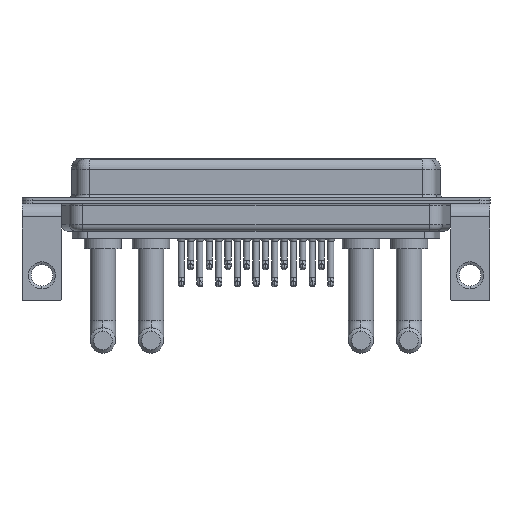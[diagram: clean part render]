
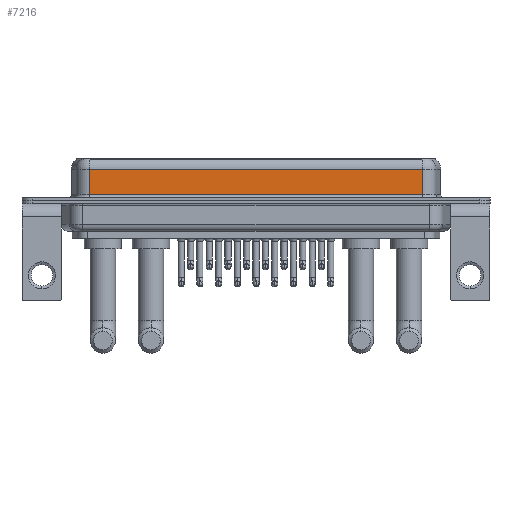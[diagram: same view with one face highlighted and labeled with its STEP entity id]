
A CAD part, front view. The second image highlights one B-rep face of the part: STEP entity #7216.
In plain terms, the highlighted planar face has unit normal (0, -1, 0).
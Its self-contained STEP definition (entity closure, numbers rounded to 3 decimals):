
#426 = EDGE_CURVE ( 'NONE', #21630, #22538, #20422, .T. ) ;
#877 = ORIENTED_EDGE ( 'NONE', *, *, #426, .T. ) ;
#1028 = VECTOR ( 'NONE', #13619, 1000. ) ;
#1091 = CARTESIAN_POINT ( 'NONE',  ( 56.462, -3.95, 6.4 ) ) ;
#1149 = LINE ( 'NONE', #15602, #1028 ) ;
#1449 = AXIS2_PLACEMENT_3D ( 'NONE', #1091, #13446, #4660 ) ;
#4433 = VECTOR ( 'NONE', #10505, 1000. ) ;
#4660 = DIRECTION ( 'NONE',  ( 0., 0., 1. ) ) ;
#4919 = EDGE_CURVE ( 'NONE', #10563, #21630, #1149, .T. ) ;
#4928 = ORIENTED_EDGE ( 'NONE', *, *, #17255, .F. ) ;
#5510 = ORIENTED_EDGE ( 'NONE', *, *, #4919, .T. ) ;
#6090 = ORIENTED_EDGE ( 'NONE', *, *, #15577, .T. ) ;
#6255 = VECTOR ( 'NONE', #6483, 1000. ) ;
#6483 = DIRECTION ( 'NONE',  ( 1., 0., 0. ) ) ;
#7216 = ADVANCED_FACE ( 'NONE', ( #20575 ), #11484, .F. ) ;
#8173 = DIRECTION ( 'NONE',  ( 0., 0., -1. ) ) ;
#8788 = VERTEX_POINT ( 'NONE', #19651 ) ;
#8938 = VECTOR ( 'NONE', #8173, 1000. ) ;
#9002 = CARTESIAN_POINT ( 'NONE',  ( 56.462, -3.95, 4.65 ) ) ;
#9912 = LINE ( 'NONE', #16959, #8938 ) ;
#10505 = DIRECTION ( 'NONE',  ( -1., 0., 0. ) ) ;
#10563 = VERTEX_POINT ( 'NONE', #21608 ) ;
#11484 = PLANE ( 'NONE',  #1449 ) ;
#13446 = DIRECTION ( 'NONE',  ( 0., 1., 0. ) ) ;
#13619 = DIRECTION ( 'NONE',  ( 0., 0., -1. ) ) ;
#14200 = LINE ( 'NONE', #9002, #4433 ) ;
#14253 = CARTESIAN_POINT ( 'NONE',  ( 56.462, -3.95, 0.9 ) ) ;
#15577 = EDGE_CURVE ( 'NONE', #8788, #10563, #14200, .T. ) ;
#15602 = CARTESIAN_POINT ( 'NONE',  ( 7.038, -3.95, 6.4 ) ) ;
#16959 = CARTESIAN_POINT ( 'NONE',  ( 56.462, -3.95, 6.4 ) ) ;
#17255 = EDGE_CURVE ( 'NONE', #8788, #22538, #9912, .T. ) ;
#18270 = EDGE_LOOP ( 'NONE', ( #4928, #6090, #5510, #877 ) ) ;
#19651 = CARTESIAN_POINT ( 'NONE',  ( 56.462, -3.95, 4.65 ) ) ;
#20422 = LINE ( 'NONE', #22267, #6255 ) ;
#20575 = FACE_OUTER_BOUND ( 'NONE', #18270, .T. ) ;
#21554 = CARTESIAN_POINT ( 'NONE',  ( 7.038, -3.95, 0.9 ) ) ;
#21608 = CARTESIAN_POINT ( 'NONE',  ( 7.038, -3.95, 4.65 ) ) ;
#21630 = VERTEX_POINT ( 'NONE', #21554 ) ;
#22267 = CARTESIAN_POINT ( 'NONE',  ( 56.462, -3.95, 0.9 ) ) ;
#22538 = VERTEX_POINT ( 'NONE', #14253 ) ;
